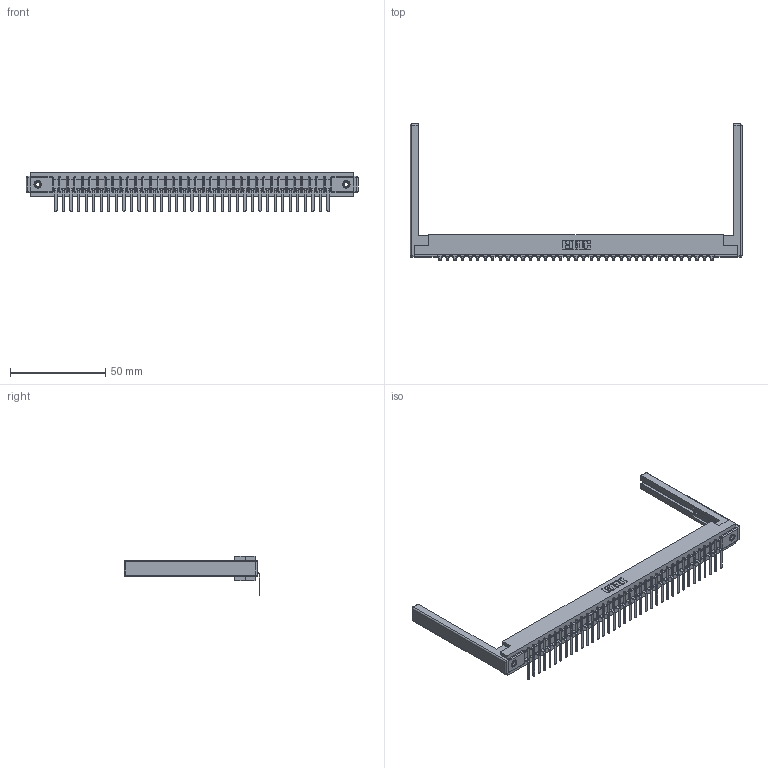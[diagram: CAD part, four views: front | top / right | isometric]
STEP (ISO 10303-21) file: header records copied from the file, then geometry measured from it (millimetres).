
FILE_DESCRIPTION (( 'STEP AP203' ), '1' );
FILE_NAME ('357-037-557-168.STEP', '2019-09-17T07:32:00', ( '' ), ( '' ), 'SwSTEP 2.0', 'SolidWorks 2016', '' );
FILE_SCHEMA (( 'CONFIG_CONTROL_DESIGN' ));
Length unit declared in the file: inch
Products named in the file (5): 307-290-002_557; 307-220-068; 307 Part_.156 Dia Mounting Holes; 345-250-001_345-250-001-102; 357-037-557-168
Assembly tree (42 placements, depth 2):
  357-037-557-168
    307 Part_.156 Dia Mounting Holes
    307-290-002_557  x37
    307-220-068  x2
    345-250-001_345-250-001-102  x2
Bounding box: 174.04 x 71.29 x 20.66 mm (x, y, z)
Volume: 23064.7 mm3; surface area: 27997 mm2
Topology: 42 solids, 42 shells, 3196 faces, 9741 edges, 6370 vertices
Faces by surface type: plane 1897, cylinder 1199, sphere 84, cone 12, torus 4
Entity records: 35949 total; most frequent: CARTESIAN_POINT 6029, ORIENTED_EDGE 6008, DIRECTION 5878, EDGE_CURVE 3004, VECTOR 2296, LINE 2296, VERTEX_POINT 1942, AXIS2_PLACEMENT_3D 1791
